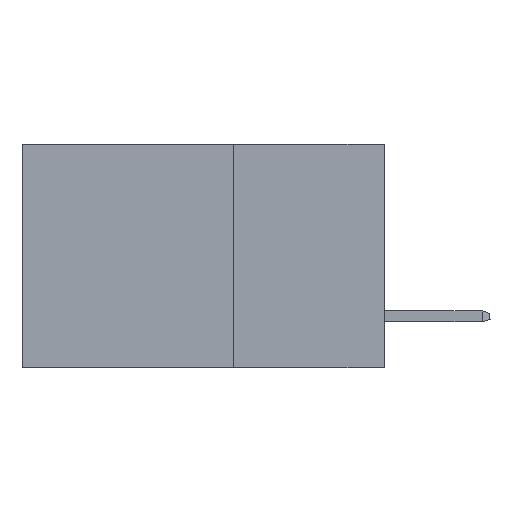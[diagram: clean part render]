
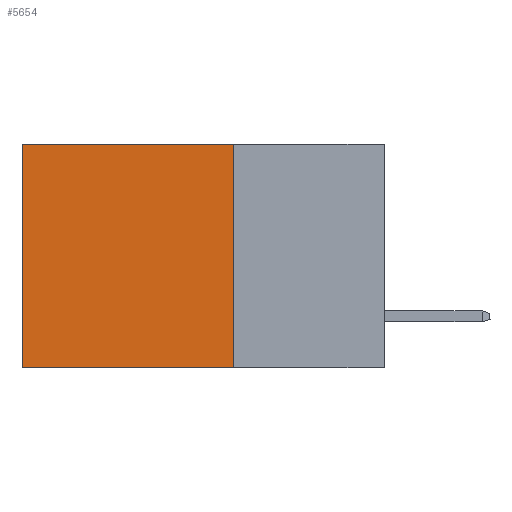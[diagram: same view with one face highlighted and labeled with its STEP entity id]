
A CAD part, left-side view. The second image highlights one B-rep face of the part: STEP entity #5654.
In plain terms, the highlighted planar face has unit normal (-1, 0, 0).
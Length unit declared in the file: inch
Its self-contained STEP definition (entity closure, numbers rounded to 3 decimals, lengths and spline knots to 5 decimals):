
#298 = LINE ( 'NONE', #8385, #12504 ) ;
#1926 = LINE ( 'NONE', #9424, #5215 ) ;
#2086 = EDGE_CURVE ( 'NONE', #7896, #3305, #3948, .T. ) ;
#2741 = PLANE ( 'NONE',  #13682 ) ;
#2840 = DIRECTION ( 'NONE',  ( 1., 0., 0. ) ) ;
#3163 = ORIENTED_EDGE ( 'NONE', *, *, #13440, .T. ) ;
#3305 = VERTEX_POINT ( 'NONE', #7314 ) ;
#3948 = LINE ( 'NONE', #9658, #10247 ) ;
#4041 = ORIENTED_EDGE ( 'NONE', *, *, #7444, .F. ) ;
#4373 = DIRECTION ( 'NONE',  ( 0., 1., 0. ) ) ;
#4483 = EDGE_LOOP ( 'NONE', ( #7441, #5874, #4041, #3163 ) ) ;
#5164 = CARTESIAN_POINT ( 'NONE',  ( 0.298, 0.25, 0. ) ) ;
#5215 = VECTOR ( 'NONE', #7176, 39.37008 ) ;
#5233 = CARTESIAN_POINT ( 'NONE',  ( 0.298, 0.25, -0.37 ) ) ;
#5467 = VERTEX_POINT ( 'NONE', #12825 ) ;
#5654 = ADVANCED_FACE ( 'NONE', ( #10075 ), #2741, .F. ) ;
#5874 = ORIENTED_EDGE ( 'NONE', *, *, #2086, .F. ) ;
#7176 = DIRECTION ( 'NONE',  ( 0., 0., -1. ) ) ;
#7314 = CARTESIAN_POINT ( 'NONE',  ( 0.298, 0.6, -0.37 ) ) ;
#7441 = ORIENTED_EDGE ( 'NONE', *, *, #12174, .T. ) ;
#7444 = EDGE_CURVE ( 'NONE', #13345, #7896, #1926, .T. ) ;
#7593 = DIRECTION ( 'NONE',  ( 0., 0., -1. ) ) ;
#7896 = VERTEX_POINT ( 'NONE', #5233 ) ;
#8385 = CARTESIAN_POINT ( 'NONE',  ( 0.298, 0.6, 0. ) ) ;
#9424 = CARTESIAN_POINT ( 'NONE',  ( 0.298, 0.25, 0. ) ) ;
#9557 = DIRECTION ( 'NONE',  ( 0., 1., 0. ) ) ;
#9575 = LINE ( 'NONE', #13857, #14423 ) ;
#9658 = CARTESIAN_POINT ( 'NONE',  ( 0.298, 0.25, -0.37 ) ) ;
#10075 = FACE_OUTER_BOUND ( 'NONE', #4483, .T. ) ;
#10247 = VECTOR ( 'NONE', #9557, 39.37008 ) ;
#11808 = DIRECTION ( 'NONE',  ( 0., 0., -1. ) ) ;
#12174 = EDGE_CURVE ( 'NONE', #5467, #3305, #298, .T. ) ;
#12504 = VECTOR ( 'NONE', #11808, 39.37008 ) ;
#12825 = CARTESIAN_POINT ( 'NONE',  ( 0.298, 0.6, 0. ) ) ;
#13345 = VERTEX_POINT ( 'NONE', #14578 ) ;
#13440 = EDGE_CURVE ( 'NONE', #13345, #5467, #9575, .T. ) ;
#13682 = AXIS2_PLACEMENT_3D ( 'NONE', #5164, #2840, #7593 ) ;
#13857 = CARTESIAN_POINT ( 'NONE',  ( 0.298, 0.25, 0. ) ) ;
#14423 = VECTOR ( 'NONE', #4373, 39.37008 ) ;
#14578 = CARTESIAN_POINT ( 'NONE',  ( 0.298, 0.25, 0. ) ) ;
